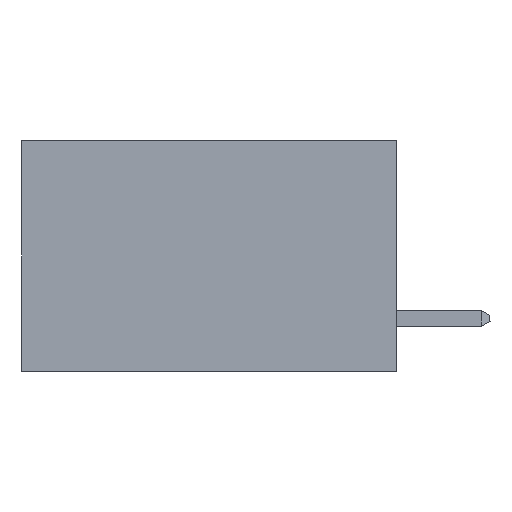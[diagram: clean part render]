
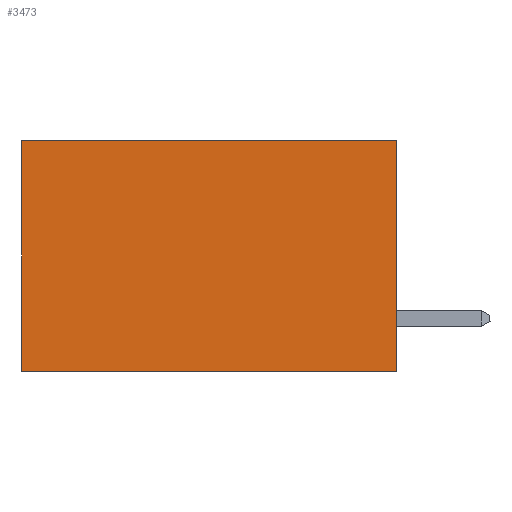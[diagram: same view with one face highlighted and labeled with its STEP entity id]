
A CAD part, left-side view. The second image highlights one B-rep face of the part: STEP entity #3473.
In plain terms, the highlighted planar face has unit normal (-1, 0, 0).
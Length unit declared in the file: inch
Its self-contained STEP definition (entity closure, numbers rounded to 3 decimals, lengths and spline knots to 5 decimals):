
#113 = VERTEX_POINT ( 'NONE', #13510 ) ;
#1135 = EDGE_CURVE ( 'NONE', #14626, #13958, #15898, .T. ) ;
#1936 = CARTESIAN_POINT ( 'NONE',  ( 0.298, 0.6, -0.37 ) ) ;
#2334 = LINE ( 'NONE', #11837, #12769 ) ;
#3317 = ORIENTED_EDGE ( 'NONE', *, *, #10590, .F. ) ;
#3473 = ADVANCED_FACE ( 'NONE', ( #7472 ), #17816, .F. ) ;
#4992 = ORIENTED_EDGE ( 'NONE', *, *, #1135, .F. ) ;
#5037 = AXIS2_PLACEMENT_3D ( 'NONE', #7791, #9380, #6253 ) ;
#5237 = CARTESIAN_POINT ( 'NONE',  ( 0.298, 0., -0.37 ) ) ;
#5245 = CARTESIAN_POINT ( 'NONE',  ( 0.298, 0., 0. ) ) ;
#6237 = VERTEX_POINT ( 'NONE', #18178 ) ;
#6253 = DIRECTION ( 'NONE',  ( 0., 0., -1. ) ) ;
#7449 = ORIENTED_EDGE ( 'NONE', *, *, #14618, .T. ) ;
#7472 = FACE_OUTER_BOUND ( 'NONE', #21380, .T. ) ;
#7558 = VECTOR ( 'NONE', #20140, 39.37008 ) ;
#7791 = CARTESIAN_POINT ( 'NONE',  ( 0.298, 0., 0. ) ) ;
#8399 = CARTESIAN_POINT ( 'NONE',  ( 0.298, 0., -0.37 ) ) ;
#8513 = ORIENTED_EDGE ( 'NONE', *, *, #10368, .T. ) ;
#9380 = DIRECTION ( 'NONE',  ( 1., 0., 0. ) ) ;
#10368 = EDGE_CURVE ( 'NONE', #6237, #113, #12701, .T. ) ;
#10590 = EDGE_CURVE ( 'NONE', #6237, #14626, #19536, .T. ) ;
#11837 = CARTESIAN_POINT ( 'NONE',  ( 0.298, 0.6, 0. ) ) ;
#12161 = CARTESIAN_POINT ( 'NONE',  ( 0.298, 0., 0. ) ) ;
#12701 = LINE ( 'NONE', #12161, #17428 ) ;
#12769 = VECTOR ( 'NONE', #13506, 39.37008 ) ;
#13506 = DIRECTION ( 'NONE',  ( 0., 0., -1. ) ) ;
#13510 = CARTESIAN_POINT ( 'NONE',  ( 0.298, 0.6, 0. ) ) ;
#13958 = VERTEX_POINT ( 'NONE', #1936 ) ;
#14618 = EDGE_CURVE ( 'NONE', #113, #13958, #2334, .T. ) ;
#14626 = VERTEX_POINT ( 'NONE', #5237 ) ;
#15898 = LINE ( 'NONE', #8399, #7558 ) ;
#16930 = DIRECTION ( 'NONE',  ( 0., 0., -1. ) ) ;
#17428 = VECTOR ( 'NONE', #20657, 39.37008 ) ;
#17816 = PLANE ( 'NONE',  #5037 ) ;
#18178 = CARTESIAN_POINT ( 'NONE',  ( 0.298, 0., 0. ) ) ;
#19536 = LINE ( 'NONE', #5245, #20061 ) ;
#20061 = VECTOR ( 'NONE', #16930, 39.37008 ) ;
#20140 = DIRECTION ( 'NONE',  ( 0., 1., 0. ) ) ;
#20657 = DIRECTION ( 'NONE',  ( 0., 1., 0. ) ) ;
#21380 = EDGE_LOOP ( 'NONE', ( #7449, #4992, #3317, #8513 ) ) ;
